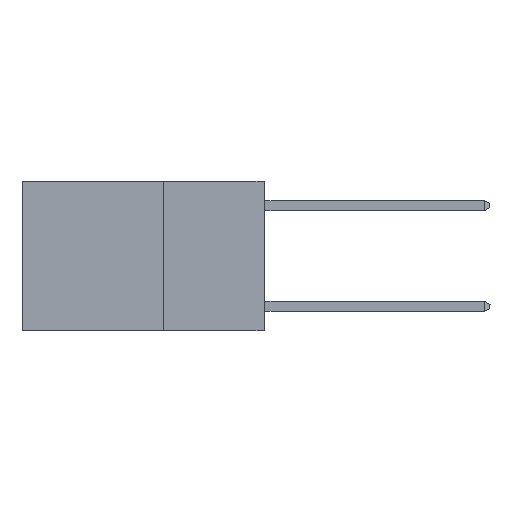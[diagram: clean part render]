
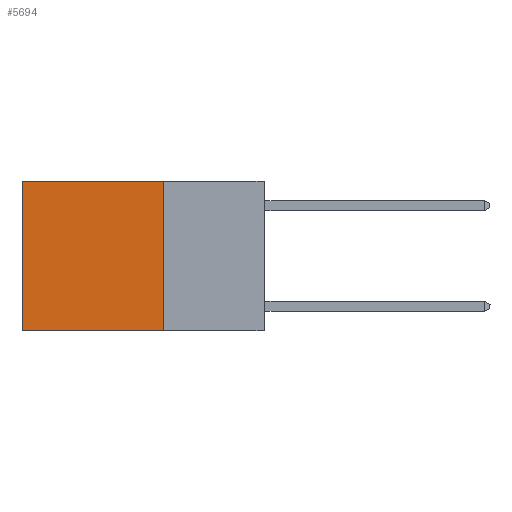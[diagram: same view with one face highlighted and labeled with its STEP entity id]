
A CAD part, left-side view. The second image highlights one B-rep face of the part: STEP entity #5694.
In plain terms, the highlighted planar face has unit normal (-1, 0, 0).
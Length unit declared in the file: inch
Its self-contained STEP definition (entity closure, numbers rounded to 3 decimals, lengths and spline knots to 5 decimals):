
#59 = CARTESIAN_POINT ( 'NONE',  ( 0.2625, 0.6, 0. ) ) ;
#186 = DIRECTION ( 'NONE',  ( 0., 1., 0. ) ) ;
#442 = LINE ( 'NONE', #11865, #5535 ) ;
#937 = DIRECTION ( 'NONE',  ( 0., 0., -1. ) ) ;
#1036 = ORIENTED_EDGE ( 'NONE', *, *, #3643, .T. ) ;
#1605 = VECTOR ( 'NONE', #2526, 39.37008 ) ;
#1676 = CARTESIAN_POINT ( 'NONE',  ( 0.2625, 0.25, 0. ) ) ;
#2526 = DIRECTION ( 'NONE',  ( 0., 0., -1. ) ) ;
#2653 = VECTOR ( 'NONE', #5142, 39.37008 ) ;
#2733 = DIRECTION ( 'NONE',  ( 0., 1., 0. ) ) ;
#3643 = EDGE_CURVE ( 'NONE', #11271, #12239, #7329, .T. ) ;
#3722 = CARTESIAN_POINT ( 'NONE',  ( 0.2625, 0.6, -0.37 ) ) ;
#4360 = ORIENTED_EDGE ( 'NONE', *, *, #7905, .F. ) ;
#4441 = VECTOR ( 'NONE', #2733, 39.37008 ) ;
#4466 = AXIS2_PLACEMENT_3D ( 'NONE', #5001, #6944, #937 ) ;
#5001 = CARTESIAN_POINT ( 'NONE',  ( 0.2625, 0.25, 0. ) ) ;
#5142 = DIRECTION ( 'NONE',  ( 0., 0., -1. ) ) ;
#5265 = EDGE_CURVE ( 'NONE', #12239, #10275, #10436, .T. ) ;
#5535 = VECTOR ( 'NONE', #186, 39.37008 ) ;
#5694 = ADVANCED_FACE ( 'NONE', ( #8184 ), #5991, .F. ) ;
#5730 = ORIENTED_EDGE ( 'NONE', *, *, #12341, .F. ) ;
#5991 = PLANE ( 'NONE',  #4466 ) ;
#6303 = EDGE_LOOP ( 'NONE', ( #11887, #5730, #4360, #1036 ) ) ;
#6944 = DIRECTION ( 'NONE',  ( 1., 0., 0. ) ) ;
#7329 = LINE ( 'NONE', #1676, #4441 ) ;
#7905 = EDGE_CURVE ( 'NONE', #11271, #11668, #9513, .T. ) ;
#8184 = FACE_OUTER_BOUND ( 'NONE', #6303, .T. ) ;
#8969 = CARTESIAN_POINT ( 'NONE',  ( 0.2625, 0.25, -0.37 ) ) ;
#9417 = CARTESIAN_POINT ( 'NONE',  ( 0.2625, 0.25, 0. ) ) ;
#9513 = LINE ( 'NONE', #9417, #1605 ) ;
#10275 = VERTEX_POINT ( 'NONE', #3722 ) ;
#10436 = LINE ( 'NONE', #10858, #2653 ) ;
#10858 = CARTESIAN_POINT ( 'NONE',  ( 0.2625, 0.6, 0. ) ) ;
#11271 = VERTEX_POINT ( 'NONE', #12039 ) ;
#11668 = VERTEX_POINT ( 'NONE', #8969 ) ;
#11865 = CARTESIAN_POINT ( 'NONE',  ( 0.2625, 0.25, -0.37 ) ) ;
#11887 = ORIENTED_EDGE ( 'NONE', *, *, #5265, .T. ) ;
#12039 = CARTESIAN_POINT ( 'NONE',  ( 0.2625, 0.25, 0. ) ) ;
#12239 = VERTEX_POINT ( 'NONE', #59 ) ;
#12341 = EDGE_CURVE ( 'NONE', #11668, #10275, #442, .T. ) ;
